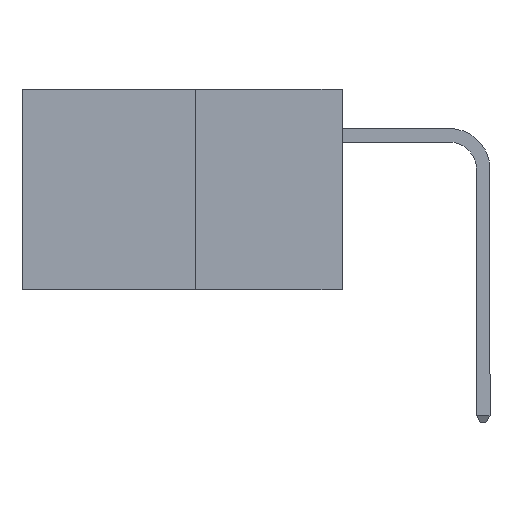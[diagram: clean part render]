
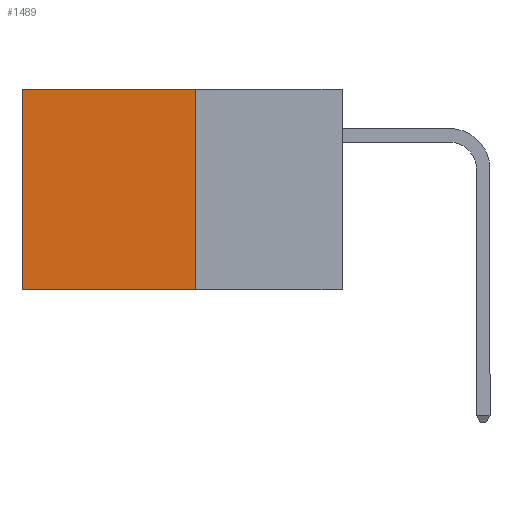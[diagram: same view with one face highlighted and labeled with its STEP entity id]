
A CAD part, left-side view. The second image highlights one B-rep face of the part: STEP entity #1489.
In plain terms, the highlighted planar face has unit normal (-1, 0, 0).
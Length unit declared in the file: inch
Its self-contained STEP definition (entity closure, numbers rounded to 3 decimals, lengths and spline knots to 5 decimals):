
#708 = LINE ( 'NONE', #28307, #20471 ) ;
#1007 = EDGE_CURVE ( 'NONE', #10098, #18182, #9172, .T. ) ;
#1371 = CARTESIAN_POINT ( 'NONE',  ( 0.277, 0.59, 0. ) ) ;
#1489 = ADVANCED_FACE ( 'NONE', ( #8146 ), #19706, .F. ) ;
#2550 = EDGE_CURVE ( 'NONE', #10098, #5980, #16211, .T. ) ;
#3081 = VECTOR ( 'NONE', #4247, 39.37008 ) ;
#4204 = CARTESIAN_POINT ( 'NONE',  ( 0.277, 0.27, 0. ) ) ;
#4247 = DIRECTION ( 'NONE',  ( 0., 0., -1. ) ) ;
#4939 = CARTESIAN_POINT ( 'NONE',  ( 0.277, 0.27, -0.37 ) ) ;
#5980 = VERTEX_POINT ( 'NONE', #1371 ) ;
#6721 = EDGE_LOOP ( 'NONE', ( #13060, #8537, #21748, #23992 ) ) ;
#7170 = LINE ( 'NONE', #11751, #18563 ) ;
#7521 = DIRECTION ( 'NONE',  ( 0., 1., 0. ) ) ;
#8146 = FACE_OUTER_BOUND ( 'NONE', #6721, .T. ) ;
#8537 = ORIENTED_EDGE ( 'NONE', *, *, #9281, .F. ) ;
#9172 = LINE ( 'NONE', #4939, #3081 ) ;
#9281 = EDGE_CURVE ( 'NONE', #18182, #25880, #708, .T. ) ;
#10098 = VERTEX_POINT ( 'NONE', #24480 ) ;
#10155 = VECTOR ( 'NONE', #7521, 39.37008 ) ;
#10818 = CARTESIAN_POINT ( 'NONE',  ( 0.277, 0.59, -0.37 ) ) ;
#11696 = EDGE_CURVE ( 'NONE', #5980, #25880, #7170, .T. ) ;
#11751 = CARTESIAN_POINT ( 'NONE',  ( 0.277, 0.59, -0.37 ) ) ;
#13060 = ORIENTED_EDGE ( 'NONE', *, *, #11696, .T. ) ;
#14607 = DIRECTION ( 'NONE',  ( 0., 1., 0. ) ) ;
#15061 = AXIS2_PLACEMENT_3D ( 'NONE', #19655, #19451, #19387 ) ;
#15352 = CARTESIAN_POINT ( 'NONE',  ( 0.277, 0.27, -0.37 ) ) ;
#16211 = LINE ( 'NONE', #4204, #10155 ) ;
#18182 = VERTEX_POINT ( 'NONE', #15352 ) ;
#18563 = VECTOR ( 'NONE', #27758, 39.37008 ) ;
#19387 = DIRECTION ( 'NONE',  ( 0., 0., -1. ) ) ;
#19451 = DIRECTION ( 'NONE',  ( 1., 0., 0. ) ) ;
#19655 = CARTESIAN_POINT ( 'NONE',  ( 0.277, 0.27, -0.37 ) ) ;
#19706 = PLANE ( 'NONE',  #15061 ) ;
#20471 = VECTOR ( 'NONE', #14607, 39.37008 ) ;
#21748 = ORIENTED_EDGE ( 'NONE', *, *, #1007, .F. ) ;
#23992 = ORIENTED_EDGE ( 'NONE', *, *, #2550, .T. ) ;
#24480 = CARTESIAN_POINT ( 'NONE',  ( 0.277, 0.27, 0. ) ) ;
#25880 = VERTEX_POINT ( 'NONE', #10818 ) ;
#27758 = DIRECTION ( 'NONE',  ( 0., 0., -1. ) ) ;
#28307 = CARTESIAN_POINT ( 'NONE',  ( 0.277, 0.27, -0.37 ) ) ;
